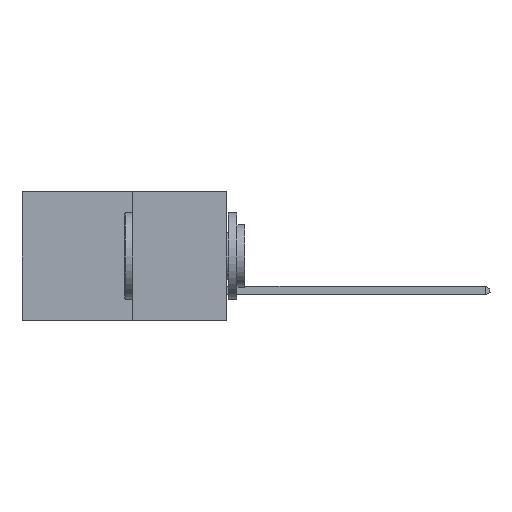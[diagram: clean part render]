
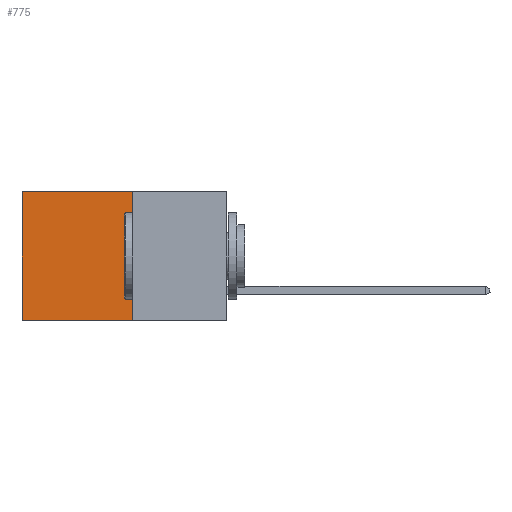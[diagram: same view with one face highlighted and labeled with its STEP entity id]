
A CAD part, left-side view. The second image highlights one B-rep face of the part: STEP entity #775.
In plain terms, the highlighted planar face has unit normal (-1, 0, 0).
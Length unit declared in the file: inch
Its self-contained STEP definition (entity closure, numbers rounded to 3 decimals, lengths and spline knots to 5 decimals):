
#488 = VECTOR ( 'NONE', #23683, 39.37008 ) ;
#617 = VECTOR ( 'NONE', #2938, 39.37008 ) ;
#775 = ADVANCED_FACE ( 'NONE', ( #18458 ), #31151, .F. ) ;
#1423 = VERTEX_POINT ( 'NONE', #22829 ) ;
#1490 = EDGE_CURVE ( 'NONE', #16009, #24473, #23849, .T. ) ;
#1575 = CARTESIAN_POINT ( 'NONE',  ( 0.277, 0.27, 0. ) ) ;
#2245 = ORIENTED_EDGE ( 'NONE', *, *, #6361, .F. ) ;
#2938 = DIRECTION ( 'NONE',  ( 0., 1., 0. ) ) ;
#3373 = EDGE_LOOP ( 'NONE', ( #7878, #2245, #31946, #30649 ) ) ;
#3658 = CARTESIAN_POINT ( 'NONE',  ( 0.277, 0.27, -0.37 ) ) ;
#6361 = EDGE_CURVE ( 'NONE', #1423, #24473, #14105, .T. ) ;
#7878 = ORIENTED_EDGE ( 'NONE', *, *, #1490, .T. ) ;
#8188 = CARTESIAN_POINT ( 'NONE',  ( 0.277, 0.59, -0.37 ) ) ;
#9812 = VERTEX_POINT ( 'NONE', #1575 ) ;
#10415 = VECTOR ( 'NONE', #22715, 39.37008 ) ;
#11526 = CARTESIAN_POINT ( 'NONE',  ( 0.277, 0.27, -0.37 ) ) ;
#13174 = EDGE_CURVE ( 'NONE', #9812, #16009, #13970, .T. ) ;
#13970 = LINE ( 'NONE', #31214, #488 ) ;
#14105 = LINE ( 'NONE', #3658, #617 ) ;
#16009 = VERTEX_POINT ( 'NONE', #16462 ) ;
#16462 = CARTESIAN_POINT ( 'NONE',  ( 0.277, 0.59, 0. ) ) ;
#16656 = EDGE_CURVE ( 'NONE', #9812, #1423, #18521, .T. ) ;
#18458 = FACE_OUTER_BOUND ( 'NONE', #3373, .T. ) ;
#18521 = LINE ( 'NONE', #11526, #26017 ) ;
#22647 = CARTESIAN_POINT ( 'NONE',  ( 0.277, 0.59, -0.37 ) ) ;
#22715 = DIRECTION ( 'NONE',  ( 0., 0., -1. ) ) ;
#22829 = CARTESIAN_POINT ( 'NONE',  ( 0.277, 0.27, -0.37 ) ) ;
#23040 = CARTESIAN_POINT ( 'NONE',  ( 0.277, 0.27, -0.37 ) ) ;
#23289 = DIRECTION ( 'NONE',  ( 1., 0., 0. ) ) ;
#23683 = DIRECTION ( 'NONE',  ( 0., 1., 0. ) ) ;
#23849 = LINE ( 'NONE', #22647, #10415 ) ;
#24473 = VERTEX_POINT ( 'NONE', #8188 ) ;
#26017 = VECTOR ( 'NONE', #26677, 39.37008 ) ;
#26677 = DIRECTION ( 'NONE',  ( 0., 0., -1. ) ) ;
#27782 = AXIS2_PLACEMENT_3D ( 'NONE', #23040, #23289, #30498 ) ;
#30498 = DIRECTION ( 'NONE',  ( 0., 0., -1. ) ) ;
#30649 = ORIENTED_EDGE ( 'NONE', *, *, #13174, .T. ) ;
#31151 = PLANE ( 'NONE',  #27782 ) ;
#31214 = CARTESIAN_POINT ( 'NONE',  ( 0.277, 0.27, 0. ) ) ;
#31946 = ORIENTED_EDGE ( 'NONE', *, *, #16656, .F. ) ;
